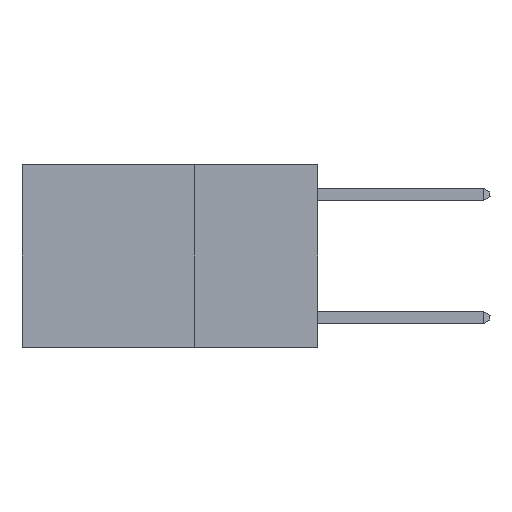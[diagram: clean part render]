
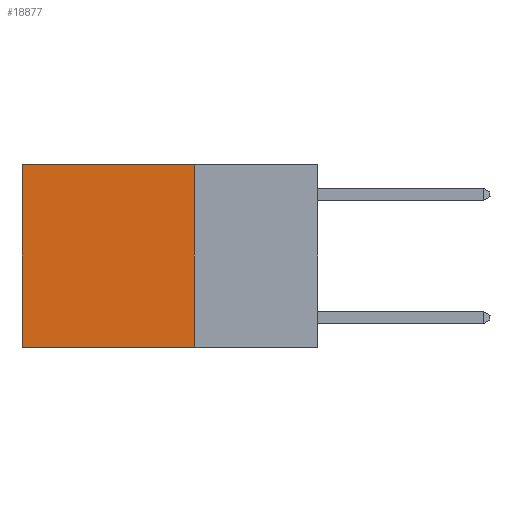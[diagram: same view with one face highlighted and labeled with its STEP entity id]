
A CAD part, left-side view. The second image highlights one B-rep face of the part: STEP entity #18877.
In plain terms, the highlighted planar face has unit normal (-1, 0, 0).
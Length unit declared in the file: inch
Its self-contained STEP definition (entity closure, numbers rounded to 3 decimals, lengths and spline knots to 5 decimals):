
#247 = ORIENTED_EDGE ( 'NONE', *, *, #6982, .T. ) ;
#893 = EDGE_CURVE ( 'NONE', #3861, #2049, #11899, .T. ) ;
#1295 = VERTEX_POINT ( 'NONE', #14468 ) ;
#1561 = FACE_OUTER_BOUND ( 'NONE', #15804, .T. ) ;
#2049 = VERTEX_POINT ( 'NONE', #18047 ) ;
#2510 = DIRECTION ( 'NONE',  ( 1., 0., 0. ) ) ;
#3070 = VECTOR ( 'NONE', #14085, 39.37008 ) ;
#3861 = VERTEX_POINT ( 'NONE', #13736 ) ;
#3948 = ORIENTED_EDGE ( 'NONE', *, *, #11740, .T. ) ;
#5011 = VECTOR ( 'NONE', #8141, 39.37008 ) ;
#5566 = VECTOR ( 'NONE', #16578, 39.37008 ) ;
#5610 = EDGE_CURVE ( 'NONE', #16670, #3861, #11615, .T. ) ;
#6234 = ORIENTED_EDGE ( 'NONE', *, *, #5610, .F. ) ;
#6982 = EDGE_CURVE ( 'NONE', #16670, #1295, #18292, .T. ) ;
#7131 = CARTESIAN_POINT ( 'NONE',  ( 0.2625, 0.25, 0. ) ) ;
#7869 = ORIENTED_EDGE ( 'NONE', *, *, #893, .F. ) ;
#8005 = CARTESIAN_POINT ( 'NONE',  ( 0.2625, 0.25, 0. ) ) ;
#8120 = VECTOR ( 'NONE', #10264, 39.37008 ) ;
#8141 = DIRECTION ( 'NONE',  ( 0., 0., -1. ) ) ;
#8746 = CARTESIAN_POINT ( 'NONE',  ( 0.2625, 0.25, 0. ) ) ;
#10264 = DIRECTION ( 'NONE',  ( 0., 0., -1. ) ) ;
#10430 = CARTESIAN_POINT ( 'NONE',  ( 0.2625, 0.25, 0. ) ) ;
#11615 = LINE ( 'NONE', #8005, #5011 ) ;
#11740 = EDGE_CURVE ( 'NONE', #1295, #2049, #18869, .T. ) ;
#11899 = LINE ( 'NONE', #17127, #3070 ) ;
#13736 = CARTESIAN_POINT ( 'NONE',  ( 0.2625, 0.25, -0.37 ) ) ;
#14085 = DIRECTION ( 'NONE',  ( 0., 1., 0. ) ) ;
#14468 = CARTESIAN_POINT ( 'NONE',  ( 0.2625, 0.6, 0. ) ) ;
#14984 = CARTESIAN_POINT ( 'NONE',  ( 0.2625, 0.6, 0. ) ) ;
#15804 = EDGE_LOOP ( 'NONE', ( #3948, #7869, #6234, #247 ) ) ;
#16578 = DIRECTION ( 'NONE',  ( 0., 1., 0. ) ) ;
#16670 = VERTEX_POINT ( 'NONE', #10430 ) ;
#17127 = CARTESIAN_POINT ( 'NONE',  ( 0.2625, 0.25, -0.37 ) ) ;
#18047 = CARTESIAN_POINT ( 'NONE',  ( 0.2625, 0.6, -0.37 ) ) ;
#18292 = LINE ( 'NONE', #7131, #5566 ) ;
#18367 = PLANE ( 'NONE',  #19361 ) ;
#18869 = LINE ( 'NONE', #14984, #8120 ) ;
#18877 = ADVANCED_FACE ( 'NONE', ( #1561 ), #18367, .F. ) ;
#19361 = AXIS2_PLACEMENT_3D ( 'NONE', #8746, #2510, #19947 ) ;
#19947 = DIRECTION ( 'NONE',  ( 0., 0., -1. ) ) ;
